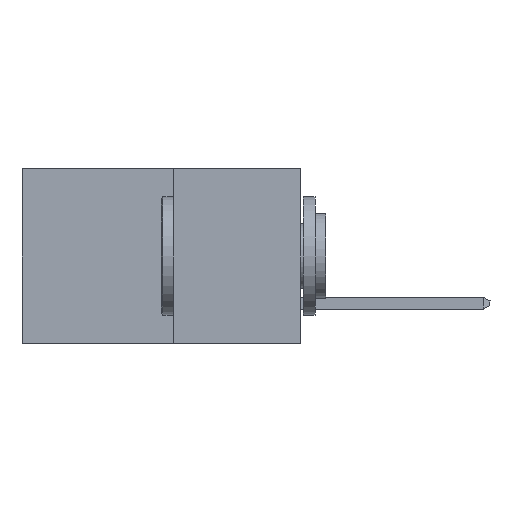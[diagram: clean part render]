
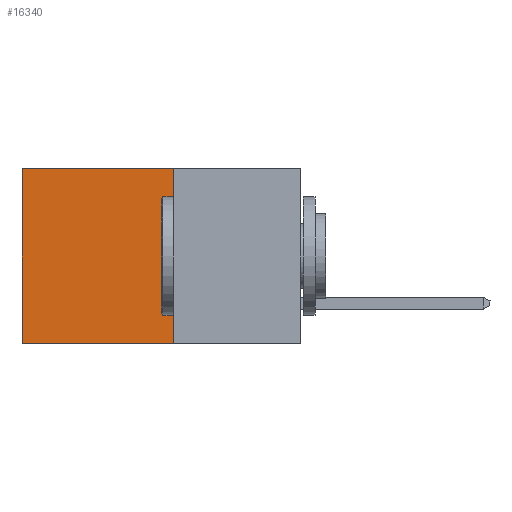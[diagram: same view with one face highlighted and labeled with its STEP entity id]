
A CAD part, left-side view. The second image highlights one B-rep face of the part: STEP entity #16340.
In plain terms, the highlighted planar face has unit normal (-1, 0, 0).
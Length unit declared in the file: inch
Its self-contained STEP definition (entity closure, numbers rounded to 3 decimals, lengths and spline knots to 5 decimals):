
#565 = VERTEX_POINT ( 'NONE', #12730 ) ;
#923 = VECTOR ( 'NONE', #12193, 39.37008 ) ;
#1039 = VECTOR ( 'NONE', #16070, 39.37008 ) ;
#1094 = CARTESIAN_POINT ( 'NONE',  ( 0.277, 0.59, -0.37 ) ) ;
#1604 = FACE_OUTER_BOUND ( 'NONE', #2988, .T. ) ;
#1728 = CARTESIAN_POINT ( 'NONE',  ( 0.277, 0.27, -0.37 ) ) ;
#2988 = EDGE_LOOP ( 'NONE', ( #8220, #7484, #5512, #14419 ) ) ;
#3470 = DIRECTION ( 'NONE',  ( 0., 0., -1. ) ) ;
#4270 = VECTOR ( 'NONE', #6659, 39.37008 ) ;
#5274 = LINE ( 'NONE', #14443, #1039 ) ;
#5512 = ORIENTED_EDGE ( 'NONE', *, *, #5709, .F. ) ;
#5709 = EDGE_CURVE ( 'NONE', #11399, #16942, #16642, .T. ) ;
#6659 = DIRECTION ( 'NONE',  ( 0., 1., 0. ) ) ;
#7484 = ORIENTED_EDGE ( 'NONE', *, *, #19700, .F. ) ;
#8220 = ORIENTED_EDGE ( 'NONE', *, *, #14821, .T. ) ;
#8238 = AXIS2_PLACEMENT_3D ( 'NONE', #9766, #12971, #3470 ) ;
#8472 = CARTESIAN_POINT ( 'NONE',  ( 0.277, 0.59, -0.37 ) ) ;
#9723 = CARTESIAN_POINT ( 'NONE',  ( 0.277, 0.27, -0.37 ) ) ;
#9766 = CARTESIAN_POINT ( 'NONE',  ( 0.277, 0.27, -0.37 ) ) ;
#10276 = DIRECTION ( 'NONE',  ( 0., 0., -1. ) ) ;
#11008 = CARTESIAN_POINT ( 'NONE',  ( 0.277, 0.27, 0. ) ) ;
#11399 = VERTEX_POINT ( 'NONE', #11008 ) ;
#12193 = DIRECTION ( 'NONE',  ( 0., 0., -1. ) ) ;
#12405 = VECTOR ( 'NONE', #10276, 39.37008 ) ;
#12703 = LINE ( 'NONE', #12934, #4270 ) ;
#12730 = CARTESIAN_POINT ( 'NONE',  ( 0.277, 0.59, 0. ) ) ;
#12934 = CARTESIAN_POINT ( 'NONE',  ( 0.277, 0.27, 0. ) ) ;
#12971 = DIRECTION ( 'NONE',  ( 1., 0., 0. ) ) ;
#13573 = LINE ( 'NONE', #1094, #923 ) ;
#14419 = ORIENTED_EDGE ( 'NONE', *, *, #19110, .T. ) ;
#14443 = CARTESIAN_POINT ( 'NONE',  ( 0.277, 0.27, -0.37 ) ) ;
#14821 = EDGE_CURVE ( 'NONE', #565, #20385, #13573, .T. ) ;
#16070 = DIRECTION ( 'NONE',  ( 0., 1., 0. ) ) ;
#16128 = PLANE ( 'NONE',  #8238 ) ;
#16340 = ADVANCED_FACE ( 'NONE', ( #1604 ), #16128, .F. ) ;
#16642 = LINE ( 'NONE', #9723, #12405 ) ;
#16942 = VERTEX_POINT ( 'NONE', #1728 ) ;
#19110 = EDGE_CURVE ( 'NONE', #11399, #565, #12703, .T. ) ;
#19700 = EDGE_CURVE ( 'NONE', #16942, #20385, #5274, .T. ) ;
#20385 = VERTEX_POINT ( 'NONE', #8472 ) ;
